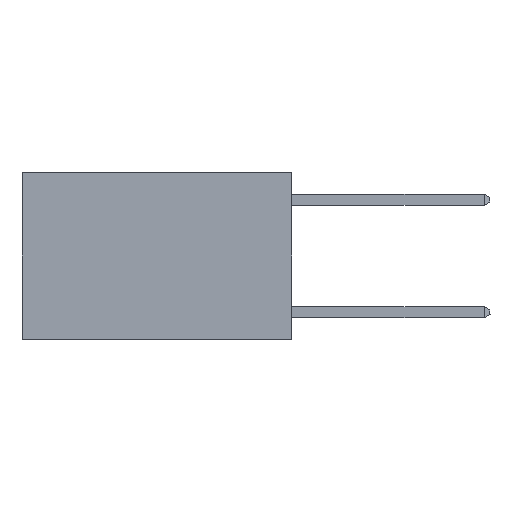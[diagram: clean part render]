
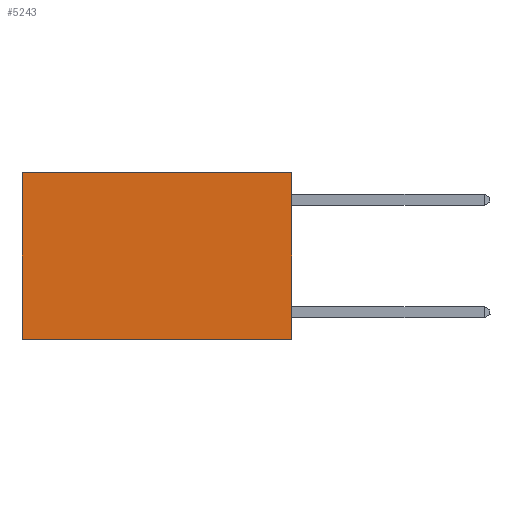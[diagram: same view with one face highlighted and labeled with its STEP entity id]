
A CAD part, left-side view. The second image highlights one B-rep face of the part: STEP entity #5243.
In plain terms, the highlighted planar face has unit normal (-1, 0, 0).
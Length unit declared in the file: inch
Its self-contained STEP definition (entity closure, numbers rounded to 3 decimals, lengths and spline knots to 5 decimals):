
#47 = DIRECTION ( 'NONE',  ( 0., 0., -1. ) ) ;
#851 = CARTESIAN_POINT ( 'NONE',  ( 0.2625, 0., 0. ) ) ;
#1087 = LINE ( 'NONE', #1823, #15917 ) ;
#1256 = DIRECTION ( 'NONE',  ( 0., 0., -1. ) ) ;
#1554 = VECTOR ( 'NONE', #2631, 39.37008 ) ;
#1700 = VERTEX_POINT ( 'NONE', #6634 ) ;
#1823 = CARTESIAN_POINT ( 'NONE',  ( 0.2625, 0., 0. ) ) ;
#2414 = VERTEX_POINT ( 'NONE', #8584 ) ;
#2631 = DIRECTION ( 'NONE',  ( 0., 0., -1. ) ) ;
#2640 = EDGE_CURVE ( 'NONE', #14752, #2414, #13603, .T. ) ;
#2875 = VECTOR ( 'NONE', #15726, 39.37008 ) ;
#3624 = EDGE_LOOP ( 'NONE', ( #10290, #13971, #7019, #17929 ) ) ;
#4058 = FACE_OUTER_BOUND ( 'NONE', #3624, .T. ) ;
#4184 = CARTESIAN_POINT ( 'NONE',  ( 0.2625, 0., 0. ) ) ;
#4808 = EDGE_CURVE ( 'NONE', #2414, #10973, #14372, .T. ) ;
#5243 = ADVANCED_FACE ( 'NONE', ( #4058 ), #17148, .F. ) ;
#6535 = AXIS2_PLACEMENT_3D ( 'NONE', #14462, #8942, #47 ) ;
#6634 = CARTESIAN_POINT ( 'NONE',  ( 0.2625, 0.6, 0. ) ) ;
#7019 = ORIENTED_EDGE ( 'NONE', *, *, #2640, .F. ) ;
#7044 = EDGE_CURVE ( 'NONE', #1700, #10973, #7561, .T. ) ;
#7122 = VECTOR ( 'NONE', #1256, 39.37008 ) ;
#7466 = CARTESIAN_POINT ( 'NONE',  ( 0.2625, 0., -0.37 ) ) ;
#7561 = LINE ( 'NONE', #14223, #7122 ) ;
#7924 = DIRECTION ( 'NONE',  ( 0., 1., 0. ) ) ;
#8584 = CARTESIAN_POINT ( 'NONE',  ( 0.2625, 0., -0.37 ) ) ;
#8942 = DIRECTION ( 'NONE',  ( 1., 0., 0. ) ) ;
#10177 = CARTESIAN_POINT ( 'NONE',  ( 0.2625, 0.6, -0.37 ) ) ;
#10290 = ORIENTED_EDGE ( 'NONE', *, *, #7044, .T. ) ;
#10973 = VERTEX_POINT ( 'NONE', #10177 ) ;
#13098 = EDGE_CURVE ( 'NONE', #14752, #1700, #1087, .T. ) ;
#13603 = LINE ( 'NONE', #4184, #1554 ) ;
#13971 = ORIENTED_EDGE ( 'NONE', *, *, #4808, .F. ) ;
#14223 = CARTESIAN_POINT ( 'NONE',  ( 0.2625, 0.6, 0. ) ) ;
#14372 = LINE ( 'NONE', #7466, #2875 ) ;
#14462 = CARTESIAN_POINT ( 'NONE',  ( 0.2625, 0., 0. ) ) ;
#14752 = VERTEX_POINT ( 'NONE', #851 ) ;
#15726 = DIRECTION ( 'NONE',  ( 0., 1., 0. ) ) ;
#15917 = VECTOR ( 'NONE', #7924, 39.37008 ) ;
#17148 = PLANE ( 'NONE',  #6535 ) ;
#17929 = ORIENTED_EDGE ( 'NONE', *, *, #13098, .T. ) ;
